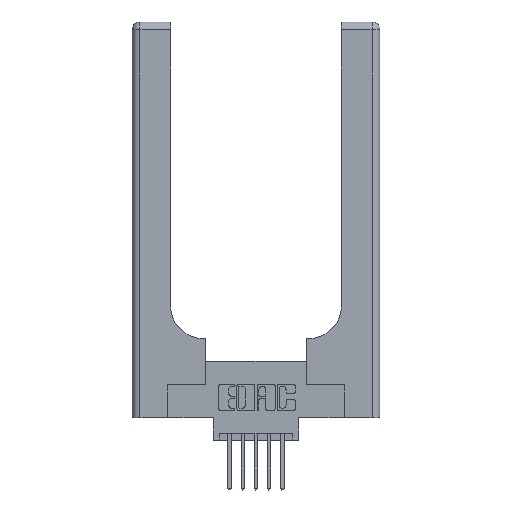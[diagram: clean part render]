
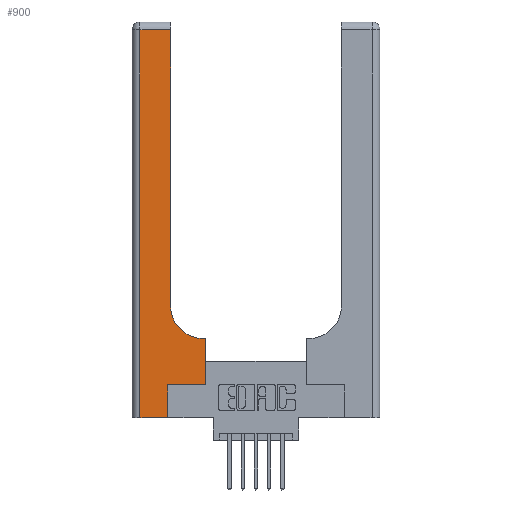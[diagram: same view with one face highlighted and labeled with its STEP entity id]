
A CAD part, top view. The second image highlights one B-rep face of the part: STEP entity #900.
In plain terms, the highlighted planar face has unit normal (0, 0, 1).
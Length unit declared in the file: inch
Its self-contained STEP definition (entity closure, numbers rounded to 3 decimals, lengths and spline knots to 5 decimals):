
#470 = ORIENTED_EDGE ( 'NONE', *, *, #6001, .T. ) ;
#652 = VERTEX_POINT ( 'NONE', #11129 ) ;
#868 = DIRECTION ( 'NONE',  ( 0., -1., 0. ) ) ;
#900 = ADVANCED_FACE ( 'NONE', ( #9327 ), #8218, .F. ) ;
#979 = DIRECTION ( 'NONE',  ( 1., 0., 0. ) ) ;
#1076 = VERTEX_POINT ( 'NONE', #7809 ) ;
#1224 = LINE ( 'NONE', #2798, #7256 ) ;
#1361 = EDGE_CURVE ( 'NONE', #12105, #9814, #12821, .T. ) ;
#1453 = EDGE_LOOP ( 'NONE', ( #8042, #2466, #8715, #470, #3952, #12559, #7218, #7886, #5360 ) ) ;
#1547 = DIRECTION ( 'NONE',  ( 0., 0., -1. ) ) ;
#1833 = AXIS2_PLACEMENT_3D ( 'NONE', #3954, #1547, #13221 ) ;
#2110 = EDGE_CURVE ( 'NONE', #9814, #5732, #6334, .T. ) ;
#2466 = ORIENTED_EDGE ( 'NONE', *, *, #2110, .T. ) ;
#2758 = DIRECTION ( 'NONE',  ( -1., 0., 0. ) ) ;
#2798 = CARTESIAN_POINT ( 'NONE',  ( 0.5585, 0.25, 0.37 ) ) ;
#3079 = VERTEX_POINT ( 'NONE', #9031 ) ;
#3572 = DIRECTION ( 'NONE',  ( 1., 0., 0. ) ) ;
#3952 = ORIENTED_EDGE ( 'NONE', *, *, #4162, .T. ) ;
#3954 = CARTESIAN_POINT ( 'NONE',  ( 0., 3., 0.37 ) ) ;
#4162 = EDGE_CURVE ( 'NONE', #652, #1076, #11309, .T. ) ;
#4326 = DIRECTION ( 'NONE',  ( 0., 1., 0. ) ) ;
#4529 = VECTOR ( 'NONE', #13382, 39.37008 ) ;
#4739 = EDGE_CURVE ( 'NONE', #5732, #3079, #11291, .T. ) ;
#5075 = EDGE_CURVE ( 'NONE', #12730, #10545, #1224, .T. ) ;
#5360 = ORIENTED_EDGE ( 'NONE', *, *, #8630, .T. ) ;
#5732 = VERTEX_POINT ( 'NONE', #6355 ) ;
#5918 = CARTESIAN_POINT ( 'NONE',  ( 0., 0., 0.37 ) ) ;
#6001 = EDGE_CURVE ( 'NONE', #3079, #652, #7420, .T. ) ;
#6305 = CARTESIAN_POINT ( 'NONE',  ( 0.2915, 0.85, 0.37 ) ) ;
#6313 = CIRCLE ( 'NONE', #11667, 0.25 ) ;
#6334 = LINE ( 'NONE', #9900, #11365 ) ;
#6355 = CARTESIAN_POINT ( 'NONE',  ( 0.06, 2.94, 0.37 ) ) ;
#6573 = CARTESIAN_POINT ( 'NONE',  ( 0.06, 3., 0.37 ) ) ;
#6654 = CARTESIAN_POINT ( 'NONE',  ( 0.5585, 0.6, 0.37 ) ) ;
#7143 = VECTOR ( 'NONE', #8236, 39.37008 ) ;
#7218 = ORIENTED_EDGE ( 'NONE', *, *, #5075, .T. ) ;
#7256 = VECTOR ( 'NONE', #9413, 39.37008 ) ;
#7420 = LINE ( 'NONE', #5918, #4529 ) ;
#7449 = CARTESIAN_POINT ( 'NONE',  ( 0.5585, 0.25, 0.37 ) ) ;
#7651 = EDGE_CURVE ( 'NONE', #1076, #12730, #10737, .T. ) ;
#7742 = DIRECTION ( 'NONE',  ( 0., 0., -1. ) ) ;
#7809 = CARTESIAN_POINT ( 'NONE',  ( 0.269, 0.25, 0.37 ) ) ;
#7886 = ORIENTED_EDGE ( 'NONE', *, *, #13309, .T. ) ;
#8042 = ORIENTED_EDGE ( 'NONE', *, *, #1361, .T. ) ;
#8218 = PLANE ( 'NONE',  #1833 ) ;
#8236 = DIRECTION ( 'NONE',  ( 0., 1., 0. ) ) ;
#8461 = VECTOR ( 'NONE', #4326, 39.37008 ) ;
#8630 = EDGE_CURVE ( 'NONE', #11232, #12105, #6313, .T. ) ;
#8715 = ORIENTED_EDGE ( 'NONE', *, *, #4739, .T. ) ;
#8857 = LINE ( 'NONE', #12994, #14185 ) ;
#9031 = CARTESIAN_POINT ( 'NONE',  ( 0.06, 0., 0.37 ) ) ;
#9268 = CARTESIAN_POINT ( 'NONE',  ( 0.2915, 3., 0.37 ) ) ;
#9327 = FACE_OUTER_BOUND ( 'NONE', #1453, .T. ) ;
#9413 = DIRECTION ( 'NONE',  ( 0., 1., 0. ) ) ;
#9717 = CARTESIAN_POINT ( 'NONE',  ( 0.269, 0., 0.37 ) ) ;
#9814 = VERTEX_POINT ( 'NONE', #13976 ) ;
#9900 = CARTESIAN_POINT ( 'NONE',  ( 0., 2.94, 0.37 ) ) ;
#10067 = VECTOR ( 'NONE', #3572, 39.37008 ) ;
#10545 = VERTEX_POINT ( 'NONE', #6654 ) ;
#10737 = LINE ( 'NONE', #12210, #10067 ) ;
#11129 = CARTESIAN_POINT ( 'NONE',  ( 0.269, 0., 0.37 ) ) ;
#11232 = VERTEX_POINT ( 'NONE', #13283 ) ;
#11291 = LINE ( 'NONE', #6573, #13432 ) ;
#11309 = LINE ( 'NONE', #9717, #8461 ) ;
#11365 = VECTOR ( 'NONE', #2758, 39.37008 ) ;
#11667 = AXIS2_PLACEMENT_3D ( 'NONE', #14123, #7742, #979 ) ;
#12105 = VERTEX_POINT ( 'NONE', #6305 ) ;
#12210 = CARTESIAN_POINT ( 'NONE',  ( 0.269, 0.25, 0.37 ) ) ;
#12559 = ORIENTED_EDGE ( 'NONE', *, *, #7651, .T. ) ;
#12730 = VERTEX_POINT ( 'NONE', #7449 ) ;
#12821 = LINE ( 'NONE', #9268, #7143 ) ;
#12994 = CARTESIAN_POINT ( 'NONE',  ( 0.2915, 0.6, 0.37 ) ) ;
#13221 = DIRECTION ( 'NONE',  ( -1., 0., 0. ) ) ;
#13283 = CARTESIAN_POINT ( 'NONE',  ( 0.5415, 0.6, 0.37 ) ) ;
#13309 = EDGE_CURVE ( 'NONE', #10545, #11232, #8857, .T. ) ;
#13382 = DIRECTION ( 'NONE',  ( 1., 0., 0. ) ) ;
#13432 = VECTOR ( 'NONE', #868, 39.37008 ) ;
#13976 = CARTESIAN_POINT ( 'NONE',  ( 0.2915, 2.94, 0.37 ) ) ;
#14048 = DIRECTION ( 'NONE',  ( -1., 0., 0. ) ) ;
#14123 = CARTESIAN_POINT ( 'NONE',  ( 0.5415, 0.85, 0.37 ) ) ;
#14185 = VECTOR ( 'NONE', #14048, 39.37008 ) ;
